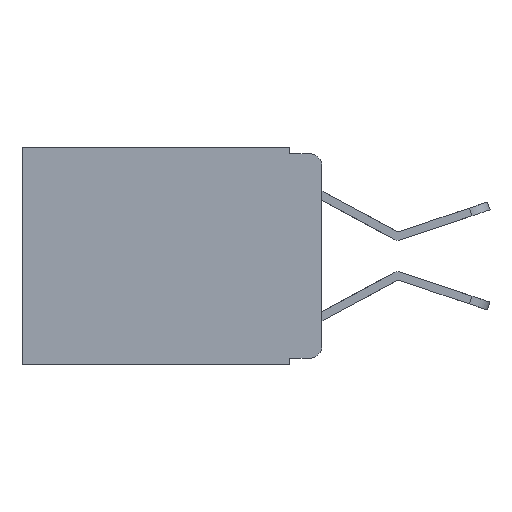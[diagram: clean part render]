
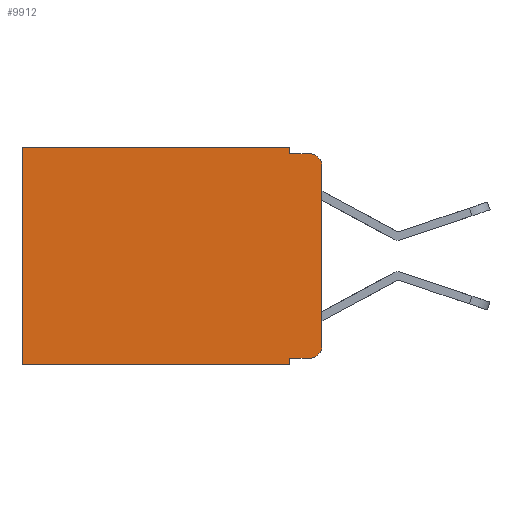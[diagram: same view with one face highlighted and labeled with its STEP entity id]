
A CAD part, left-side view. The second image highlights one B-rep face of the part: STEP entity #9912.
In plain terms, the highlighted planar face has unit normal (-1, 0, 0).
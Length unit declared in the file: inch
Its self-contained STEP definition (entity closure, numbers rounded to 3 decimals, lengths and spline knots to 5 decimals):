
#65 = CARTESIAN_POINT ( 'NONE',  ( 0.298, 0.051, -0.01 ) ) ;
#135 = CARTESIAN_POINT ( 'NONE',  ( 0.298, 0.473, 0. ) ) ;
#223 = VERTEX_POINT ( 'NONE', #135 ) ;
#323 = VERTEX_POINT ( 'NONE', #65 ) ;
#326 = DIRECTION ( 'NONE',  ( 0., 1., 0. ) ) ;
#515 = CARTESIAN_POINT ( 'NONE',  ( 0.298, 0.02, -0.03 ) ) ;
#549 = VERTEX_POINT ( 'NONE', #9293 ) ;
#592 = ORIENTED_EDGE ( 'NONE', *, *, #8460, .F. ) ;
#1113 = EDGE_LOOP ( 'NONE', ( #7924, #2954, #2394, #3701, #10124, #8185, #592, #5294, #4444, #4256 ) ) ;
#1221 = VECTOR ( 'NONE', #9174, 39.37008 ) ;
#1600 = CARTESIAN_POINT ( 'NONE',  ( 0.298, 0., 0. ) ) ;
#1670 = DIRECTION ( 'NONE',  ( 0., 0., -1. ) ) ;
#1756 = LINE ( 'NONE', #4838, #8002 ) ;
#2075 = VECTOR ( 'NONE', #7113, 39.37008 ) ;
#2119 = EDGE_CURVE ( 'NONE', #3523, #4683, #9287, .T. ) ;
#2194 = EDGE_CURVE ( 'NONE', #4452, #2490, #8379, .T. ) ;
#2249 = EDGE_CURVE ( 'NONE', #4452, #3523, #3347, .T. ) ;
#2394 = ORIENTED_EDGE ( 'NONE', *, *, #5751, .F. ) ;
#2490 = VERTEX_POINT ( 'NONE', #10046 ) ;
#2526 = DIRECTION ( 'NONE',  ( -1., 0., 0. ) ) ;
#2766 = CARTESIAN_POINT ( 'NONE',  ( 0.298, 0.051, -0.01 ) ) ;
#2884 = DIRECTION ( 'NONE',  ( 0., -1., 0. ) ) ;
#2954 = ORIENTED_EDGE ( 'NONE', *, *, #5678, .T. ) ;
#3347 = LINE ( 'NONE', #9983, #7646 ) ;
#3472 = VECTOR ( 'NONE', #4802, 39.37008 ) ;
#3523 = VERTEX_POINT ( 'NONE', #5371 ) ;
#3621 = EDGE_CURVE ( 'NONE', #549, #223, #6687, .T. ) ;
#3701 = ORIENTED_EDGE ( 'NONE', *, *, #4710, .F. ) ;
#4157 = AXIS2_PLACEMENT_3D ( 'NONE', #515, #7158, #1670 ) ;
#4256 = ORIENTED_EDGE ( 'NONE', *, *, #2119, .T. ) ;
#4444 = ORIENTED_EDGE ( 'NONE', *, *, #2249, .T. ) ;
#4452 = VERTEX_POINT ( 'NONE', #8342 ) ;
#4544 = CARTESIAN_POINT ( 'NONE',  ( 0.298, 0., -0.313 ) ) ;
#4658 = AXIS2_PLACEMENT_3D ( 'NONE', #4941, #10381, #5805 ) ;
#4683 = VERTEX_POINT ( 'NONE', #4544 ) ;
#4703 = DIRECTION ( 'NONE',  ( 0., -1., 0. ) ) ;
#4710 = EDGE_CURVE ( 'NONE', #549, #323, #7958, .T. ) ;
#4712 = VERTEX_POINT ( 'NONE', #5478 ) ;
#4802 = DIRECTION ( 'NONE',  ( 0., 0., -1. ) ) ;
#4838 = CARTESIAN_POINT ( 'NONE',  ( 0.298, 0.473, 0. ) ) ;
#4941 = CARTESIAN_POINT ( 'NONE',  ( 0.298, 0., 0. ) ) ;
#5283 = EDGE_CURVE ( 'NONE', #223, #9101, #1756, .T. ) ;
#5294 = ORIENTED_EDGE ( 'NONE', *, *, #2194, .F. ) ;
#5371 = CARTESIAN_POINT ( 'NONE',  ( 0.298, 0.02, -0.333 ) ) ;
#5478 = CARTESIAN_POINT ( 'NONE',  ( 0.298, 0., -0.03 ) ) ;
#5510 = VECTOR ( 'NONE', #4703, 39.37008 ) ;
#5579 = CARTESIAN_POINT ( 'NONE',  ( 0.298, 0.02, -0.01 ) ) ;
#5674 = DIRECTION ( 'NONE',  ( 0., 0., -1. ) ) ;
#5678 = EDGE_CURVE ( 'NONE', #4712, #11256, #9885, .T. ) ;
#5751 = EDGE_CURVE ( 'NONE', #323, #11256, #7890, .T. ) ;
#5805 = DIRECTION ( 'NONE',  ( 0., 0., -1. ) ) ;
#5877 = VECTOR ( 'NONE', #10826, 39.37008 ) ;
#6120 = CARTESIAN_POINT ( 'NONE',  ( 0.298, 0.051, 0. ) ) ;
#6285 = FACE_OUTER_BOUND ( 'NONE', #1113, .T. ) ;
#6333 = EDGE_CURVE ( 'NONE', #4712, #4683, #9507, .T. ) ;
#6687 = LINE ( 'NONE', #1600, #2075 ) ;
#7113 = DIRECTION ( 'NONE',  ( 0., 1., 0. ) ) ;
#7158 = DIRECTION ( 'NONE',  ( -1., 0., 0. ) ) ;
#7632 = AXIS2_PLACEMENT_3D ( 'NONE', #10011, #2526, #8543 ) ;
#7634 = LINE ( 'NONE', #10731, #9379 ) ;
#7646 = VECTOR ( 'NONE', #2884, 39.37008 ) ;
#7857 = CARTESIAN_POINT ( 'NONE',  ( 0.298, 0.051, 0. ) ) ;
#7890 = LINE ( 'NONE', #2766, #5510 ) ;
#7924 = ORIENTED_EDGE ( 'NONE', *, *, #6333, .F. ) ;
#7958 = LINE ( 'NONE', #7857, #5877 ) ;
#8002 = VECTOR ( 'NONE', #5674, 39.37008 ) ;
#8185 = ORIENTED_EDGE ( 'NONE', *, *, #5283, .T. ) ;
#8342 = CARTESIAN_POINT ( 'NONE',  ( 0.298, 0.051, -0.333 ) ) ;
#8379 = LINE ( 'NONE', #6120, #1221 ) ;
#8460 = EDGE_CURVE ( 'NONE', #2490, #9101, #7634, .T. ) ;
#8543 = DIRECTION ( 'NONE',  ( 0., 0., -1. ) ) ;
#9101 = VERTEX_POINT ( 'NONE', #9659 ) ;
#9174 = DIRECTION ( 'NONE',  ( 0., 0., -1. ) ) ;
#9287 = CIRCLE ( 'NONE', #7632, 0.02 ) ;
#9293 = CARTESIAN_POINT ( 'NONE',  ( 0.298, 0.051, 0. ) ) ;
#9379 = VECTOR ( 'NONE', #326, 39.37008 ) ;
#9507 = LINE ( 'NONE', #9536, #3472 ) ;
#9536 = CARTESIAN_POINT ( 'NONE',  ( 0.298, 0., 0. ) ) ;
#9649 = PLANE ( 'NONE',  #4658 ) ;
#9659 = CARTESIAN_POINT ( 'NONE',  ( 0.298, 0.473, -0.343 ) ) ;
#9885 = CIRCLE ( 'NONE', #4157, 0.02 ) ;
#9912 = ADVANCED_FACE ( 'NONE', ( #6285 ), #9649, .F. ) ;
#9983 = CARTESIAN_POINT ( 'NONE',  ( 0.298, 0.051, -0.333 ) ) ;
#10011 = CARTESIAN_POINT ( 'NONE',  ( 0.298, 0.02, -0.313 ) ) ;
#10046 = CARTESIAN_POINT ( 'NONE',  ( 0.298, 0.051, -0.343 ) ) ;
#10124 = ORIENTED_EDGE ( 'NONE', *, *, #3621, .T. ) ;
#10381 = DIRECTION ( 'NONE',  ( 1., 0., 0. ) ) ;
#10731 = CARTESIAN_POINT ( 'NONE',  ( 0.298, 0., -0.343 ) ) ;
#10826 = DIRECTION ( 'NONE',  ( 0., 0., -1. ) ) ;
#11256 = VERTEX_POINT ( 'NONE', #5579 ) ;
